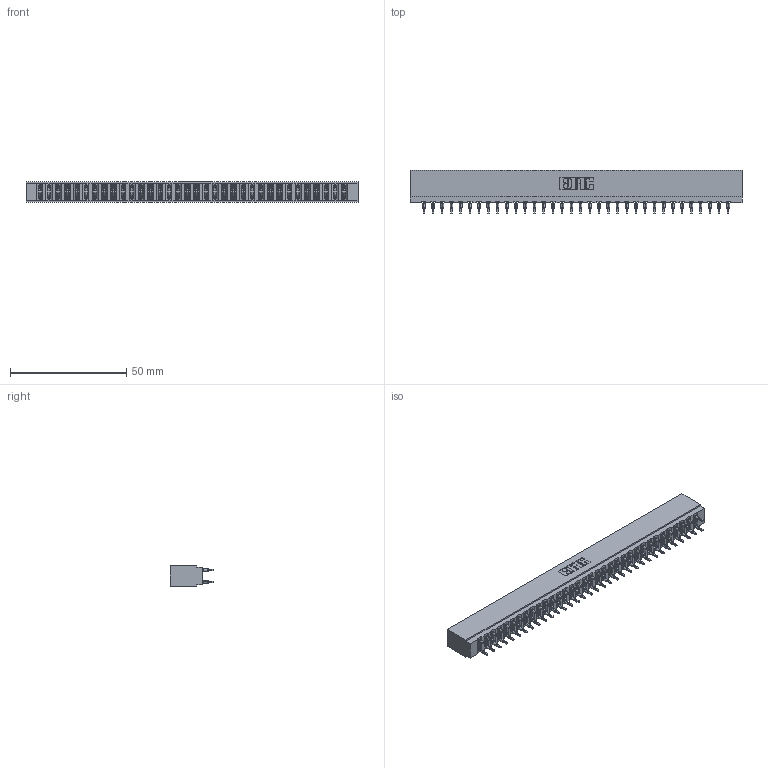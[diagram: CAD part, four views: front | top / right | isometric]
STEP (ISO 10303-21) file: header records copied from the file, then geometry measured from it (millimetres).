
FILE_DESCRIPTION (( 'STEP AP203' ), '1' );
FILE_NAME ('717-068-560-201.STEP', '2026-02-20T18:58:42', ( '' ), ( '' ), 'SwSTEP 2.0', 'SolidWorks 2023', '' );
FILE_SCHEMA (( 'CONFIG_CONTROL_DESIGN' ));
Length unit declared in the file: millimetre
Products named in the file (3): 745-292-001_560; 717-068-560-201; 717 Part_Insulator Option - 06
Assembly tree (69 placements, depth 2):
  717-068-560-201
    717 Part_Insulator Option - 06
    745-292-001_560  x68
Bounding box: 142.6 x 18.78 x 8.89 mm (x, y, z)
Volume: 12640.3 mm3; surface area: 20425.4 mm2
Topology: 69 solids, 69 shells, 6826 faces, 18679 edges, 11862 vertices
Faces by surface type: plane 3556, cylinder 1502, bspline 1360, torus 408
Entity records: 59708 total; most frequent: CARTESIAN_POINT 10871, ORIENTED_EDGE 10290, DIRECTION 8995, EDGE_CURVE 5145, VECTOR 4751, LINE 4751, VERTEX_POINT 3286, AXIS2_PLACEMENT_3D 2122
